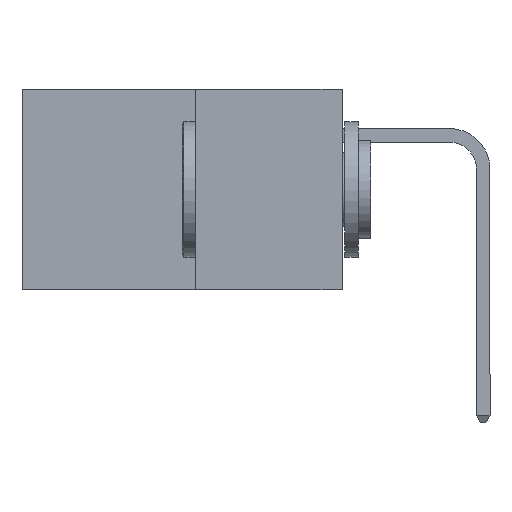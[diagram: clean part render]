
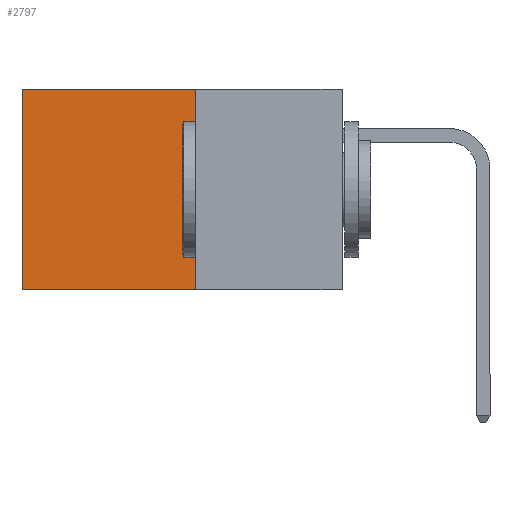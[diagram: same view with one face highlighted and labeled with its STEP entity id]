
A CAD part, left-side view. The second image highlights one B-rep face of the part: STEP entity #2797.
In plain terms, the highlighted planar face has unit normal (-1, 0, 0).
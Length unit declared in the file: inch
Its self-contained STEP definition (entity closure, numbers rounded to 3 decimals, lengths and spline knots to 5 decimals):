
#31 = EDGE_LOOP ( 'NONE', ( #325, #8153, #2514, #6784 ) ) ;
#187 = EDGE_CURVE ( 'NONE', #2704, #4808, #7117, .T. ) ;
#325 = ORIENTED_EDGE ( 'NONE', *, *, #2101, .T. ) ;
#346 = DIRECTION ( 'NONE',  ( 1., 0., 0. ) ) ;
#426 = VECTOR ( 'NONE', #7785, 39.37008 ) ;
#834 = DIRECTION ( 'NONE',  ( 0., 1., 0. ) ) ;
#1069 = VERTEX_POINT ( 'NONE', #2596 ) ;
#1540 = DIRECTION ( 'NONE',  ( 0., 0., -1. ) ) ;
#1628 = VERTEX_POINT ( 'NONE', #4777 ) ;
#2101 = EDGE_CURVE ( 'NONE', #1628, #1069, #3569, .T. ) ;
#2290 = CARTESIAN_POINT ( 'NONE',  ( 0.277, 0.27, 0. ) ) ;
#2514 = ORIENTED_EDGE ( 'NONE', *, *, #187, .F. ) ;
#2596 = CARTESIAN_POINT ( 'NONE',  ( 0.277, 0.59, -0.37 ) ) ;
#2704 = VERTEX_POINT ( 'NONE', #2706 ) ;
#2706 = CARTESIAN_POINT ( 'NONE',  ( 0.277, 0.27, 0. ) ) ;
#2797 = ADVANCED_FACE ( 'NONE', ( #5650 ), #4726, .F. ) ;
#2885 = AXIS2_PLACEMENT_3D ( 'NONE', #5306, #346, #1540 ) ;
#3033 = CARTESIAN_POINT ( 'NONE',  ( 0.277, 0.27, -0.37 ) ) ;
#3084 = CARTESIAN_POINT ( 'NONE',  ( 0.277, 0.27, -0.37 ) ) ;
#3569 = LINE ( 'NONE', #5018, #8272 ) ;
#4273 = DIRECTION ( 'NONE',  ( 0., 0., -1. ) ) ;
#4659 = EDGE_CURVE ( 'NONE', #2704, #1628, #7733, .T. ) ;
#4726 = PLANE ( 'NONE',  #2885 ) ;
#4777 = CARTESIAN_POINT ( 'NONE',  ( 0.277, 0.59, 0. ) ) ;
#4808 = VERTEX_POINT ( 'NONE', #3084 ) ;
#5018 = CARTESIAN_POINT ( 'NONE',  ( 0.277, 0.59, -0.37 ) ) ;
#5306 = CARTESIAN_POINT ( 'NONE',  ( 0.277, 0.27, -0.37 ) ) ;
#5524 = VECTOR ( 'NONE', #4273, 39.37008 ) ;
#5650 = FACE_OUTER_BOUND ( 'NONE', #31, .T. ) ;
#6278 = EDGE_CURVE ( 'NONE', #4808, #1069, #7367, .T. ) ;
#6784 = ORIENTED_EDGE ( 'NONE', *, *, #4659, .T. ) ;
#7117 = LINE ( 'NONE', #3033, #5524 ) ;
#7346 = CARTESIAN_POINT ( 'NONE',  ( 0.277, 0.27, -0.37 ) ) ;
#7367 = LINE ( 'NONE', #7346, #426 ) ;
#7554 = VECTOR ( 'NONE', #834, 39.37008 ) ;
#7661 = DIRECTION ( 'NONE',  ( 0., 0., -1. ) ) ;
#7733 = LINE ( 'NONE', #2290, #7554 ) ;
#7785 = DIRECTION ( 'NONE',  ( 0., 1., 0. ) ) ;
#8153 = ORIENTED_EDGE ( 'NONE', *, *, #6278, .F. ) ;
#8272 = VECTOR ( 'NONE', #7661, 39.37008 ) ;
